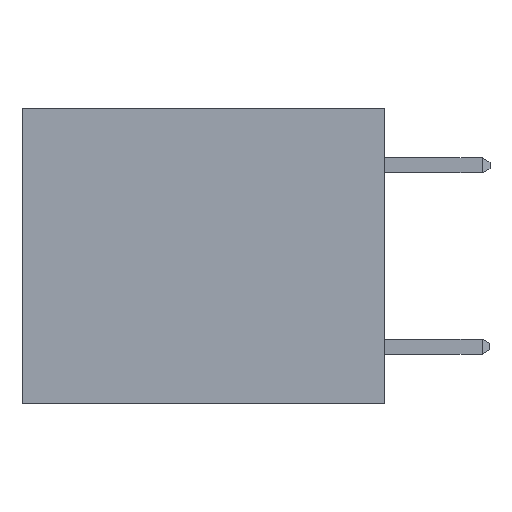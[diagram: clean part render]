
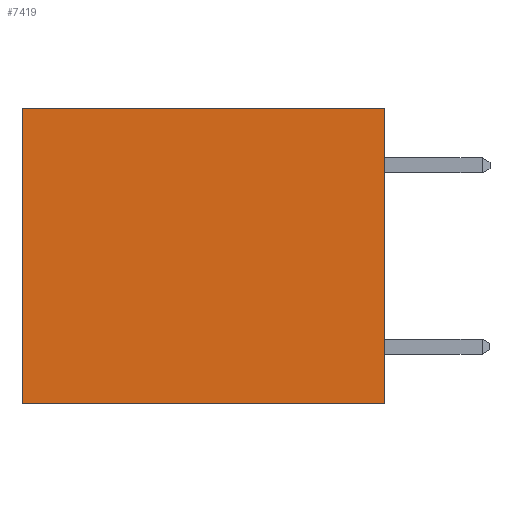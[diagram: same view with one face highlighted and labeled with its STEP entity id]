
A CAD part, left-side view. The second image highlights one B-rep face of the part: STEP entity #7419.
In plain terms, the highlighted planar face has unit normal (-1, 0, 0).
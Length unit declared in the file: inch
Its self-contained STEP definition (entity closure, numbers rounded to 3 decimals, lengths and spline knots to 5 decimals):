
#6 = DIRECTION ( 'NONE',  ( 0., 0., -1. ) ) ;
#58 = DIRECTION ( 'NONE',  ( 0., 0., -1. ) ) ;
#152 = LINE ( 'NONE', #3865, #8608 ) ;
#560 = ORIENTED_EDGE ( 'NONE', *, *, #7338, .T. ) ;
#718 = PLANE ( 'NONE',  #6887 ) ;
#766 = DIRECTION ( 'NONE',  ( 0., 0., -1. ) ) ;
#1820 = VERTEX_POINT ( 'NONE', #6835 ) ;
#2251 = CARTESIAN_POINT ( 'NONE',  ( 0.3165, 0.6, 0. ) ) ;
#2895 = ORIENTED_EDGE ( 'NONE', *, *, #4219, .F. ) ;
#3161 = VERTEX_POINT ( 'NONE', #2251 ) ;
#3606 = LINE ( 'NONE', #5575, #9870 ) ;
#3865 = CARTESIAN_POINT ( 'NONE',  ( 0.3165, 0., -0.49 ) ) ;
#3964 = EDGE_LOOP ( 'NONE', ( #560, #2895, #9719, #5797 ) ) ;
#4219 = EDGE_CURVE ( 'NONE', #10261, #1820, #152, .T. ) ;
#4286 = EDGE_CURVE ( 'NONE', #6063, #10261, #7874, .T. ) ;
#4779 = CARTESIAN_POINT ( 'NONE',  ( 0.3165, 0., -0.49 ) ) ;
#5088 = DIRECTION ( 'NONE',  ( 0., 1., 0. ) ) ;
#5404 = DIRECTION ( 'NONE',  ( 0., 1., 0. ) ) ;
#5575 = CARTESIAN_POINT ( 'NONE',  ( 0.3165, 0.6, -0.49 ) ) ;
#5797 = ORIENTED_EDGE ( 'NONE', *, *, #6034, .T. ) ;
#6034 = EDGE_CURVE ( 'NONE', #6063, #3161, #8198, .T. ) ;
#6063 = VERTEX_POINT ( 'NONE', #9401 ) ;
#6492 = FACE_OUTER_BOUND ( 'NONE', #3964, .T. ) ;
#6722 = VECTOR ( 'NONE', #5088, 39.37008 ) ;
#6835 = CARTESIAN_POINT ( 'NONE',  ( 0.3165, 0.6, -0.49 ) ) ;
#6887 = AXIS2_PLACEMENT_3D ( 'NONE', #8727, #7978, #58 ) ;
#7338 = EDGE_CURVE ( 'NONE', #3161, #1820, #3606, .T. ) ;
#7419 = ADVANCED_FACE ( 'NONE', ( #6492 ), #718, .F. ) ;
#7874 = LINE ( 'NONE', #4779, #9750 ) ;
#7978 = DIRECTION ( 'NONE',  ( 1., 0., 0. ) ) ;
#8043 = CARTESIAN_POINT ( 'NONE',  ( 0.3165, 0., -0.49 ) ) ;
#8198 = LINE ( 'NONE', #9002, #6722 ) ;
#8608 = VECTOR ( 'NONE', #5404, 39.37008 ) ;
#8727 = CARTESIAN_POINT ( 'NONE',  ( 0.3165, 0., -0.49 ) ) ;
#9002 = CARTESIAN_POINT ( 'NONE',  ( 0.3165, 0., 0. ) ) ;
#9401 = CARTESIAN_POINT ( 'NONE',  ( 0.3165, 0., 0. ) ) ;
#9719 = ORIENTED_EDGE ( 'NONE', *, *, #4286, .F. ) ;
#9750 = VECTOR ( 'NONE', #6, 39.37008 ) ;
#9870 = VECTOR ( 'NONE', #766, 39.37008 ) ;
#10261 = VERTEX_POINT ( 'NONE', #8043 ) ;
